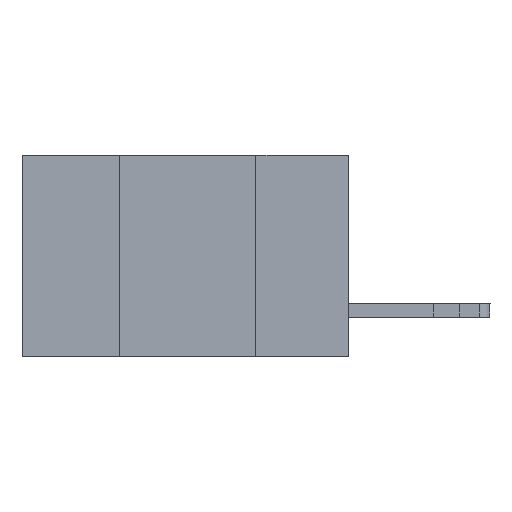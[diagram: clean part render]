
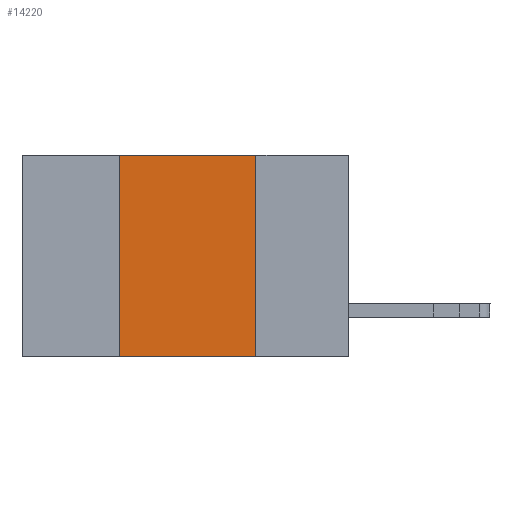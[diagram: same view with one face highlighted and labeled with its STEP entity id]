
A CAD part, left-side view. The second image highlights one B-rep face of the part: STEP entity #14220.
In plain terms, the highlighted planar face has unit normal (-1, 0, 0).
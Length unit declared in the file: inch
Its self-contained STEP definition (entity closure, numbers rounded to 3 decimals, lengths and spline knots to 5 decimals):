
#1574 = DIRECTION ( 'NONE',  ( 0., 0., 1. ) ) ;
#1817 = CARTESIAN_POINT ( 'NONE',  ( 0., 0.17, 0. ) ) ;
#2436 = CARTESIAN_POINT ( 'NONE',  ( 0., 0.17, 0. ) ) ;
#3122 = ORIENTED_EDGE ( 'NONE', *, *, #8838, .F. ) ;
#3359 = CARTESIAN_POINT ( 'NONE',  ( 0., 0.17, -0.37 ) ) ;
#3620 = CARTESIAN_POINT ( 'NONE',  ( 0., 0.6, -0.37 ) ) ;
#4183 = ORIENTED_EDGE ( 'NONE', *, *, #12952, .F. ) ;
#5605 = LINE ( 'NONE', #16089, #9240 ) ;
#5740 = PLANE ( 'NONE',  #11889 ) ;
#5753 = VECTOR ( 'NONE', #1574, 39.37008 ) ;
#6310 = VERTEX_POINT ( 'NONE', #6594 ) ;
#6313 = VERTEX_POINT ( 'NONE', #3359 ) ;
#6594 = CARTESIAN_POINT ( 'NONE',  ( 0., 0.42, 0. ) ) ;
#6739 = DIRECTION ( 'NONE',  ( 0., 0., -1. ) ) ;
#7323 = LINE ( 'NONE', #16190, #5753 ) ;
#7571 = ORIENTED_EDGE ( 'NONE', *, *, #13170, .T. ) ;
#8502 = DIRECTION ( 'NONE',  ( 0., 0., -1. ) ) ;
#8533 = LINE ( 'NONE', #2436, #10809 ) ;
#8838 = EDGE_CURVE ( 'NONE', #18039, #6313, #8533, .T. ) ;
#8867 = EDGE_LOOP ( 'NONE', ( #3122, #16995, #4183, #7571 ) ) ;
#9163 = LINE ( 'NONE', #3620, #11594 ) ;
#9240 = VECTOR ( 'NONE', #11462, 39.37008 ) ;
#10172 = VERTEX_POINT ( 'NONE', #16254 ) ;
#10809 = VECTOR ( 'NONE', #6739, 39.37008 ) ;
#11462 = DIRECTION ( 'NONE',  ( 0., -1., 0. ) ) ;
#11594 = VECTOR ( 'NONE', #15232, 39.37008 ) ;
#11596 = CARTESIAN_POINT ( 'NONE',  ( 0., 0.6, 0. ) ) ;
#11797 = DIRECTION ( 'NONE',  ( 1., 0., 0. ) ) ;
#11889 = AXIS2_PLACEMENT_3D ( 'NONE', #11596, #11797, #8502 ) ;
#12952 = EDGE_CURVE ( 'NONE', #10172, #6310, #7323, .T. ) ;
#13170 = EDGE_CURVE ( 'NONE', #10172, #6313, #9163, .T. ) ;
#14220 = ADVANCED_FACE ( 'NONE', ( #18920 ), #5740, .F. ) ;
#15232 = DIRECTION ( 'NONE',  ( 0., -1., 0. ) ) ;
#16089 = CARTESIAN_POINT ( 'NONE',  ( 0., 0.6, 0. ) ) ;
#16190 = CARTESIAN_POINT ( 'NONE',  ( 0., 0.42, 0. ) ) ;
#16254 = CARTESIAN_POINT ( 'NONE',  ( 0., 0.42, -0.37 ) ) ;
#16946 = EDGE_CURVE ( 'NONE', #6310, #18039, #5605, .T. ) ;
#16995 = ORIENTED_EDGE ( 'NONE', *, *, #16946, .F. ) ;
#18039 = VERTEX_POINT ( 'NONE', #1817 ) ;
#18920 = FACE_OUTER_BOUND ( 'NONE', #8867, .T. ) ;
